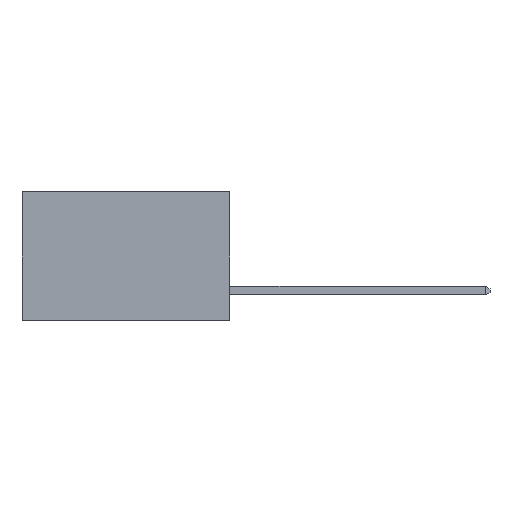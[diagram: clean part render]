
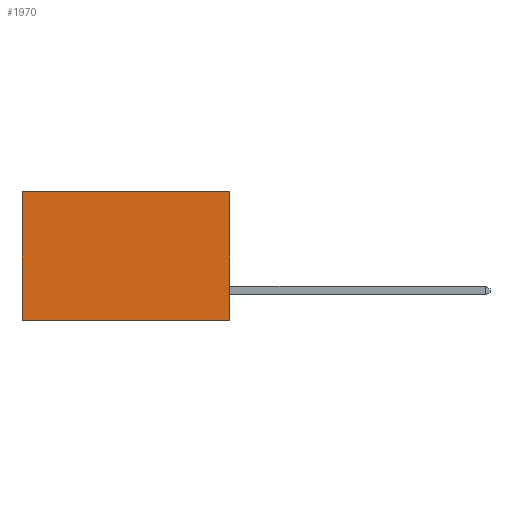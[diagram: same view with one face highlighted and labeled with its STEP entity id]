
A CAD part, left-side view. The second image highlights one B-rep face of the part: STEP entity #1970.
In plain terms, the highlighted planar face has unit normal (-1, 0, 0).
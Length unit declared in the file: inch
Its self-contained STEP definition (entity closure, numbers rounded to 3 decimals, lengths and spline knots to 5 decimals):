
#43 = FACE_OUTER_BOUND ( 'NONE', #2853, .T. ) ;
#135 = LINE ( 'NONE', #6057, #4284 ) ;
#742 = DIRECTION ( 'NONE',  ( 0., 0., -1. ) ) ;
#1332 = VERTEX_POINT ( 'NONE', #8721 ) ;
#1696 = EDGE_CURVE ( 'NONE', #1332, #1876, #8486, .T. ) ;
#1876 = VERTEX_POINT ( 'NONE', #9695 ) ;
#1970 = ADVANCED_FACE ( 'NONE', ( #43 ), #4226, .F. ) ;
#1993 = ORIENTED_EDGE ( 'NONE', *, *, #1696, .F. ) ;
#2423 = CARTESIAN_POINT ( 'NONE',  ( 0.2615, 0., -0.37 ) ) ;
#2435 = VECTOR ( 'NONE', #4355, 39.37008 ) ;
#2451 = VERTEX_POINT ( 'NONE', #2966 ) ;
#2512 = VECTOR ( 'NONE', #742, 39.37008 ) ;
#2686 = VECTOR ( 'NONE', #8457, 39.37008 ) ;
#2853 = EDGE_LOOP ( 'NONE', ( #3817, #1993, #4044, #6039 ) ) ;
#2862 = EDGE_CURVE ( 'NONE', #2451, #1332, #4527, .T. ) ;
#2966 = CARTESIAN_POINT ( 'NONE',  ( 0.2615, 0., 0. ) ) ;
#3817 = ORIENTED_EDGE ( 'NONE', *, *, #9348, .T. ) ;
#4036 = EDGE_CURVE ( 'NONE', #2451, #4185, #135, .T. ) ;
#4044 = ORIENTED_EDGE ( 'NONE', *, *, #2862, .F. ) ;
#4077 = DIRECTION ( 'NONE',  ( 1., 0., 0. ) ) ;
#4153 = DIRECTION ( 'NONE',  ( 0., 0., -1. ) ) ;
#4185 = VERTEX_POINT ( 'NONE', #4796 ) ;
#4226 = PLANE ( 'NONE',  #6491 ) ;
#4284 = VECTOR ( 'NONE', #6033, 39.37008 ) ;
#4355 = DIRECTION ( 'NONE',  ( 0., 1., 0. ) ) ;
#4438 = CARTESIAN_POINT ( 'NONE',  ( 0.2615, 0., -0.37 ) ) ;
#4527 = LINE ( 'NONE', #8251, #2512 ) ;
#4796 = CARTESIAN_POINT ( 'NONE',  ( 0.2615, 0.6, 0. ) ) ;
#6033 = DIRECTION ( 'NONE',  ( 0., 1., 0. ) ) ;
#6039 = ORIENTED_EDGE ( 'NONE', *, *, #4036, .T. ) ;
#6057 = CARTESIAN_POINT ( 'NONE',  ( 0.2615, 0., 0. ) ) ;
#6491 = AXIS2_PLACEMENT_3D ( 'NONE', #2423, #4077, #4153 ) ;
#7795 = CARTESIAN_POINT ( 'NONE',  ( 0.2615, 0.6, -0.37 ) ) ;
#8251 = CARTESIAN_POINT ( 'NONE',  ( 0.2615, 0., -0.37 ) ) ;
#8457 = DIRECTION ( 'NONE',  ( 0., 0., -1. ) ) ;
#8486 = LINE ( 'NONE', #4438, #2435 ) ;
#8504 = LINE ( 'NONE', #7795, #2686 ) ;
#8721 = CARTESIAN_POINT ( 'NONE',  ( 0.2615, 0., -0.37 ) ) ;
#9348 = EDGE_CURVE ( 'NONE', #4185, #1876, #8504, .T. ) ;
#9695 = CARTESIAN_POINT ( 'NONE',  ( 0.2615, 0.6, -0.37 ) ) ;
